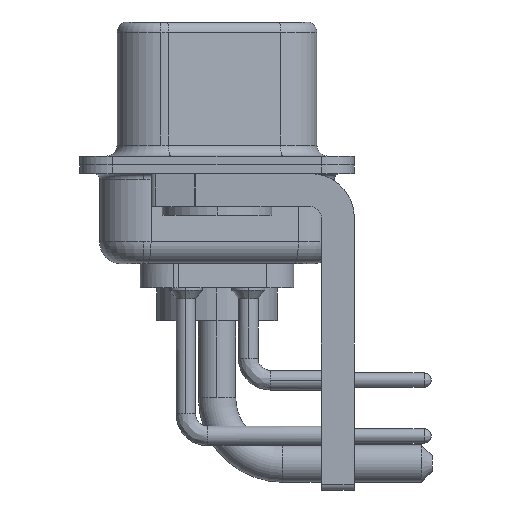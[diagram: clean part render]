
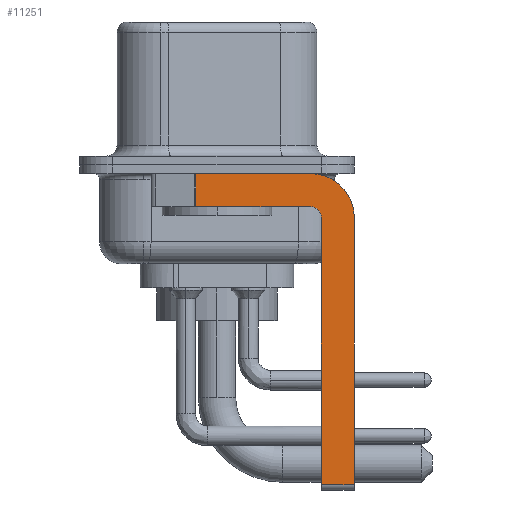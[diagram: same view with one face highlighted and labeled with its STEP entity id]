
A CAD part, left-side view. The second image highlights one B-rep face of the part: STEP entity #11251.
In plain terms, the highlighted planar face has unit normal (-1, 0, 0).
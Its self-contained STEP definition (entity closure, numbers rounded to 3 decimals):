
#231 = ORIENTED_EDGE ( 'NONE', *, *, #2690, .F. ) ;
#474 = VERTEX_POINT ( 'NONE', #8090 ) ;
#1039 = CARTESIAN_POINT ( 'NONE',  ( -2.9, -4.25, -0.4 ) ) ;
#1927 = LINE ( 'NONE', #11009, #12360 ) ;
#2075 = VECTOR ( 'NONE', #17584, 1000. ) ;
#2218 = LINE ( 'NONE', #8437, #9121 ) ;
#2496 = VERTEX_POINT ( 'NONE', #11460 ) ;
#2690 = EDGE_CURVE ( 'NONE', #7776, #11397, #19745, .T. ) ;
#3361 = CIRCLE ( 'NONE', #5938, 0.5 ) ;
#3549 = DIRECTION ( 'NONE',  ( 0., 0., -1. ) ) ;
#3915 = DIRECTION ( 'NONE',  ( 0., 0., -1. ) ) ;
#4092 = EDGE_CURVE ( 'NONE', #14923, #16491, #9887, .T. ) ;
#4310 = DIRECTION ( 'NONE',  ( 0., -1., 0. ) ) ;
#5938 = AXIS2_PLACEMENT_3D ( 'NONE', #10911, #16868, #17065 ) ;
#6400 = CARTESIAN_POINT ( 'NONE',  ( -2.9, -6.25, -2.4 ) ) ;
#7453 = LINE ( 'NONE', #9097, #7560 ) ;
#7494 = CARTESIAN_POINT ( 'NONE',  ( -2.9, 0.978, -1.9 ) ) ;
#7560 = VECTOR ( 'NONE', #4310, 1000. ) ;
#7632 = EDGE_CURVE ( 'NONE', #16334, #14047, #2218, .T. ) ;
#7776 = VERTEX_POINT ( 'NONE', #1039 ) ;
#8090 = CARTESIAN_POINT ( 'NONE',  ( -2.9, -6.25, -14.55 ) ) ;
#8437 = CARTESIAN_POINT ( 'NONE',  ( -2.9, -4.75, -14.8 ) ) ;
#8548 = CARTESIAN_POINT ( 'NONE',  ( -2.9, -4.75, -2.4 ) ) ;
#9046 = AXIS2_PLACEMENT_3D ( 'NONE', #19756, #10427, #3915 ) ;
#9097 = CARTESIAN_POINT ( 'NONE',  ( -2.9, 3., -0.4 ) ) ;
#9121 = VECTOR ( 'NONE', #11204, 1000. ) ;
#9284 = VECTOR ( 'NONE', #12824, 1000. ) ;
#9346 = EDGE_CURVE ( 'NONE', #14923, #7776, #7453, .T. ) ;
#9565 = LINE ( 'NONE', #6400, #13728 ) ;
#9669 = ORIENTED_EDGE ( 'NONE', *, *, #11039, .T. ) ;
#9887 = LINE ( 'NONE', #19113, #9284 ) ;
#9891 = EDGE_CURVE ( 'NONE', #14047, #2496, #3361, .T. ) ;
#10427 = DIRECTION ( 'NONE',  ( 1., 0., 0. ) ) ;
#10911 = CARTESIAN_POINT ( 'NONE',  ( -2.9, -4.25, -2.4 ) ) ;
#11009 = CARTESIAN_POINT ( 'NONE',  ( -2.9, -4.25, -1.9 ) ) ;
#11039 = EDGE_CURVE ( 'NONE', #16334, #474, #11419, .T. ) ;
#11204 = DIRECTION ( 'NONE',  ( 0., 0., 1. ) ) ;
#11251 = ADVANCED_FACE ( 'NONE', ( #19331 ), #18306, .F. ) ;
#11275 = ORIENTED_EDGE ( 'NONE', *, *, #7632, .F. ) ;
#11311 = CARTESIAN_POINT ( 'NONE',  ( -2.9, -4.25, -14.55 ) ) ;
#11397 = VERTEX_POINT ( 'NONE', #20110 ) ;
#11419 = LINE ( 'NONE', #11311, #2075 ) ;
#11460 = CARTESIAN_POINT ( 'NONE',  ( -2.9, -4.25, -1.9 ) ) ;
#11677 = EDGE_LOOP ( 'NONE', ( #11788, #15655, #18325, #19259, #11275, #9669, #17478, #231 ) ) ;
#11788 = ORIENTED_EDGE ( 'NONE', *, *, #9346, .F. ) ;
#12360 = VECTOR ( 'NONE', #12620, 1000. ) ;
#12482 = AXIS2_PLACEMENT_3D ( 'NONE', #15531, #20018, #14025 ) ;
#12620 = DIRECTION ( 'NONE',  ( 0., 1., 0. ) ) ;
#12824 = DIRECTION ( 'NONE',  ( 0., 0., -1. ) ) ;
#13728 = VECTOR ( 'NONE', #3549, 1000. ) ;
#14025 = DIRECTION ( 'NONE',  ( 0., 0., -1. ) ) ;
#14047 = VERTEX_POINT ( 'NONE', #8548 ) ;
#14923 = VERTEX_POINT ( 'NONE', #17651 ) ;
#15531 = CARTESIAN_POINT ( 'NONE',  ( -2.9, -4.25, -2.4 ) ) ;
#15636 = EDGE_CURVE ( 'NONE', #2496, #16491, #1927, .T. ) ;
#15655 = ORIENTED_EDGE ( 'NONE', *, *, #4092, .T. ) ;
#16334 = VERTEX_POINT ( 'NONE', #17981 ) ;
#16491 = VERTEX_POINT ( 'NONE', #7494 ) ;
#16868 = DIRECTION ( 'NONE',  ( -1., 0., 0. ) ) ;
#17065 = DIRECTION ( 'NONE',  ( 0., 0., 1. ) ) ;
#17466 = EDGE_CURVE ( 'NONE', #11397, #474, #9565, .T. ) ;
#17478 = ORIENTED_EDGE ( 'NONE', *, *, #17466, .F. ) ;
#17584 = DIRECTION ( 'NONE',  ( 0., -1., 0. ) ) ;
#17651 = CARTESIAN_POINT ( 'NONE',  ( -2.9, 0.978, -0.4 ) ) ;
#17981 = CARTESIAN_POINT ( 'NONE',  ( -2.9, -4.75, -14.55 ) ) ;
#18306 = PLANE ( 'NONE',  #12482 ) ;
#18325 = ORIENTED_EDGE ( 'NONE', *, *, #15636, .F. ) ;
#19113 = CARTESIAN_POINT ( 'NONE',  ( -2.9, 0.978, -1.9 ) ) ;
#19259 = ORIENTED_EDGE ( 'NONE', *, *, #9891, .F. ) ;
#19331 = FACE_OUTER_BOUND ( 'NONE', #11677, .T. ) ;
#19745 = CIRCLE ( 'NONE', #9046, 2. ) ;
#19756 = CARTESIAN_POINT ( 'NONE',  ( -2.9, -4.25, -2.4 ) ) ;
#20018 = DIRECTION ( 'NONE',  ( 1., 0., 0. ) ) ;
#20110 = CARTESIAN_POINT ( 'NONE',  ( -2.9, -6.25, -2.4 ) ) ;
